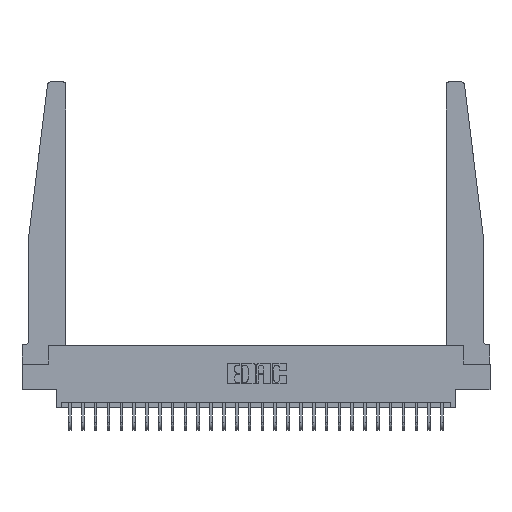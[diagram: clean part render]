
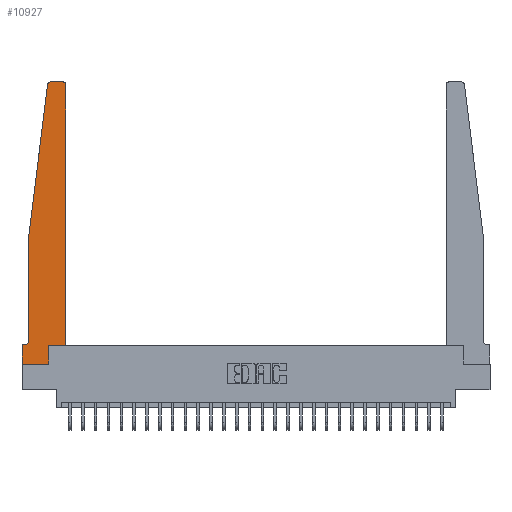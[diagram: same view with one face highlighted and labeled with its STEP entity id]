
A CAD part, top view. The second image highlights one B-rep face of the part: STEP entity #10927.
In plain terms, the highlighted planar face has unit normal (0, 0, 1).
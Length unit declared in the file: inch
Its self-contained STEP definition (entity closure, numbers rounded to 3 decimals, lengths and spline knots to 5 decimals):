
#53 = VERTEX_POINT ( 'NONE', #26011 ) ;
#137 = VERTEX_POINT ( 'NONE', #17653 ) ;
#1219 = VECTOR ( 'NONE', #7749, 39.37008 ) ;
#1226 = VERTEX_POINT ( 'NONE', #22857 ) ;
#1598 = VERTEX_POINT ( 'NONE', #12067 ) ;
#2231 = LINE ( 'NONE', #4086, #17629 ) ;
#2307 = CARTESIAN_POINT ( 'NONE',  ( 0.015, 0.1875, 0.37 ) ) ;
#2978 = CIRCLE ( 'NONE', #25849, 0.05 ) ;
#3392 = PLANE ( 'NONE',  #9828 ) ;
#3404 = VERTEX_POINT ( 'NONE', #27301 ) ;
#3586 = EDGE_CURVE ( 'NONE', #22999, #1226, #22368, .T. ) ;
#3600 = DIRECTION ( 'NONE',  ( 1., 0., 0. ) ) ;
#3619 = VECTOR ( 'NONE', #23617, 39.37008 ) ;
#3697 = LINE ( 'NONE', #27326, #1219 ) ;
#3800 = DIRECTION ( 'NONE',  ( -1., 0., 0. ) ) ;
#3836 = LINE ( 'NONE', #14809, #3619 ) ;
#4086 = CARTESIAN_POINT ( 'NONE',  ( 0.425, 0.18, 0.37 ) ) ;
#4185 = VECTOR ( 'NONE', #24917, 39.37008 ) ;
#4528 = ORIENTED_EDGE ( 'NONE', *, *, #15000, .T. ) ;
#4631 = EDGE_CURVE ( 'NONE', #18367, #1598, #27826, .T. ) ;
#5697 = DIRECTION ( 'NONE',  ( 1., 0., 0. ) ) ;
#6067 = ORIENTED_EDGE ( 'NONE', *, *, #6815, .T. ) ;
#6091 = CARTESIAN_POINT ( 'NONE',  ( 0.395, 2.75, 0.37 ) ) ;
#6325 = AXIS2_PLACEMENT_3D ( 'NONE', #9249, #24589, #13372 ) ;
#6461 = VERTEX_POINT ( 'NONE', #2307 ) ;
#6753 = CARTESIAN_POINT ( 'NONE',  ( 0.425, 2.72, 0.37 ) ) ;
#6815 = EDGE_CURVE ( 'NONE', #137, #22999, #3836, .T. ) ;
#7121 = EDGE_CURVE ( 'NONE', #6461, #137, #12481, .T. ) ;
#7220 = CIRCLE ( 'NONE', #18136, 0.03 ) ;
#7537 = VECTOR ( 'NONE', #11433, 39.37008 ) ;
#7749 = DIRECTION ( 'NONE',  ( 0., -1., 0. ) ) ;
#7797 = CARTESIAN_POINT ( 'NONE',  ( 0.395, 2.72, 0.37 ) ) ;
#7861 = CARTESIAN_POINT ( 'NONE',  ( 0.065, 0.1875, 0.37 ) ) ;
#7934 = DIRECTION ( 'NONE',  ( 0., 1., 0. ) ) ;
#8219 = EDGE_CURVE ( 'NONE', #14300, #6461, #2978, .T. ) ;
#9249 = CARTESIAN_POINT ( 'NONE',  ( 0.27653, 2.72, 0.37 ) ) ;
#9493 = EDGE_CURVE ( 'NONE', #19675, #53, #26091, .T. ) ;
#9828 = AXIS2_PLACEMENT_3D ( 'NONE', #12099, #16811, #5697 ) ;
#10927 = ADVANCED_FACE ( 'NONE', ( #16672 ), #3392, .T. ) ;
#10933 = DIRECTION ( 'NONE',  ( 0., 1., 0. ) ) ;
#10955 = VECTOR ( 'NONE', #7934, 39.37008 ) ;
#11401 = DIRECTION ( 'NONE',  ( -1., 0., 0. ) ) ;
#11433 = DIRECTION ( 'NONE',  ( 1., 0., 0. ) ) ;
#12067 = CARTESIAN_POINT ( 'NONE',  ( 0.27653, 2.75, 0.37 ) ) ;
#12099 = CARTESIAN_POINT ( 'NONE',  ( 0., 0.1875, 0.37 ) ) ;
#12148 = VECTOR ( 'NONE', #15430, 39.37008 ) ;
#12254 = CARTESIAN_POINT ( 'NONE',  ( 0.065, 0.2375, 0.37 ) ) ;
#12349 = ORIENTED_EDGE ( 'NONE', *, *, #27936, .T. ) ;
#12481 = LINE ( 'NONE', #7861, #19610 ) ;
#12694 = ORIENTED_EDGE ( 'NONE', *, *, #3586, .T. ) ;
#13372 = DIRECTION ( 'NONE',  ( 1., 0., 0. ) ) ;
#13546 = CARTESIAN_POINT ( 'NONE',  ( 0.015, 0.2375, 0.37 ) ) ;
#14006 = VERTEX_POINT ( 'NONE', #6753 ) ;
#14189 = LINE ( 'NONE', #16471, #10955 ) ;
#14300 = VERTEX_POINT ( 'NONE', #12254 ) ;
#14666 = ORIENTED_EDGE ( 'NONE', *, *, #20721, .T. ) ;
#14809 = CARTESIAN_POINT ( 'NONE',  ( 0., 0., 0.37 ) ) ;
#14932 = CIRCLE ( 'NONE', #6325, 0.03 ) ;
#15000 = EDGE_CURVE ( 'NONE', #3404, #14006, #2231, .T. ) ;
#15244 = ORIENTED_EDGE ( 'NONE', *, *, #24694, .T. ) ;
#15430 = DIRECTION ( 'NONE',  ( -0.122, -0.992, 0. ) ) ;
#16471 = CARTESIAN_POINT ( 'NONE',  ( 0.2605, 0.18, 0.37 ) ) ;
#16672 = FACE_OUTER_BOUND ( 'NONE', #23894, .T. ) ;
#16811 = DIRECTION ( 'NONE',  ( 0., 0., 1. ) ) ;
#17629 = VECTOR ( 'NONE', #10933, 39.37008 ) ;
#17653 = CARTESIAN_POINT ( 'NONE',  ( 0., 0.1875, 0.37 ) ) ;
#17884 = ORIENTED_EDGE ( 'NONE', *, *, #7121, .T. ) ;
#17987 = CARTESIAN_POINT ( 'NONE',  ( 0.425, 0.18, 0.37 ) ) ;
#18136 = AXIS2_PLACEMENT_3D ( 'NONE', #7797, #23231, #3600 ) ;
#18280 = CARTESIAN_POINT ( 'NONE',  ( 0.25, 2.75, 0.37 ) ) ;
#18291 = DIRECTION ( 'NONE',  ( 1., 0., 0. ) ) ;
#18367 = VERTEX_POINT ( 'NONE', #6091 ) ;
#18896 = ORIENTED_EDGE ( 'NONE', *, *, #4631, .T. ) ;
#19088 = EDGE_CURVE ( 'NONE', #14006, #18367, #7220, .T. ) ;
#19610 = VECTOR ( 'NONE', #3800, 39.37008 ) ;
#19675 = VERTEX_POINT ( 'NONE', #21165 ) ;
#20721 = EDGE_CURVE ( 'NONE', #25146, #3404, #22792, .T. ) ;
#21055 = CARTESIAN_POINT ( 'NONE',  ( 0., 0., 0.37 ) ) ;
#21165 = CARTESIAN_POINT ( 'NONE',  ( 0.24675, 2.72367, 0.37 ) ) ;
#21844 = CARTESIAN_POINT ( 'NONE',  ( 0.2605, 0.18, 0.37 ) ) ;
#22337 = DIRECTION ( 'NONE',  ( 0., 0., -1. ) ) ;
#22368 = LINE ( 'NONE', #26369, #7537 ) ;
#22792 = LINE ( 'NONE', #17987, #25986 ) ;
#22857 = CARTESIAN_POINT ( 'NONE',  ( 0.2605, 0., 0.37 ) ) ;
#22999 = VERTEX_POINT ( 'NONE', #21055 ) ;
#23231 = DIRECTION ( 'NONE',  ( 0., 0., 1. ) ) ;
#23617 = DIRECTION ( 'NONE',  ( 0., -1., 0. ) ) ;
#23661 = EDGE_CURVE ( 'NONE', #1598, #19675, #14932, .T. ) ;
#23894 = EDGE_LOOP ( 'NONE', ( #18896, #28144, #24222, #15244, #28203, #17884, #6067, #12694, #12349, #14666, #4528, #24949 ) ) ;
#24222 = ORIENTED_EDGE ( 'NONE', *, *, #9493, .T. ) ;
#24589 = DIRECTION ( 'NONE',  ( 0., 0., 1. ) ) ;
#24694 = EDGE_CURVE ( 'NONE', #53, #14300, #3697, .T. ) ;
#24917 = DIRECTION ( 'NONE',  ( -1., 0., 0. ) ) ;
#24949 = ORIENTED_EDGE ( 'NONE', *, *, #19088, .T. ) ;
#25146 = VERTEX_POINT ( 'NONE', #21844 ) ;
#25849 = AXIS2_PLACEMENT_3D ( 'NONE', #13546, #22337, #11401 ) ;
#25986 = VECTOR ( 'NONE', #18291, 39.37008 ) ;
#26011 = CARTESIAN_POINT ( 'NONE',  ( 0.065, 1.25, 0.37 ) ) ;
#26091 = LINE ( 'NONE', #28230, #12148 ) ;
#26369 = CARTESIAN_POINT ( 'NONE',  ( 0., 0., 0.37 ) ) ;
#27301 = CARTESIAN_POINT ( 'NONE',  ( 0.425, 0.18, 0.37 ) ) ;
#27326 = CARTESIAN_POINT ( 'NONE',  ( 0.065, 1.25, 0.37 ) ) ;
#27826 = LINE ( 'NONE', #18280, #4185 ) ;
#27936 = EDGE_CURVE ( 'NONE', #1226, #25146, #14189, .T. ) ;
#28144 = ORIENTED_EDGE ( 'NONE', *, *, #23661, .T. ) ;
#28203 = ORIENTED_EDGE ( 'NONE', *, *, #8219, .T. ) ;
#28230 = CARTESIAN_POINT ( 'NONE',  ( 0.065, 1.25, 0.37 ) ) ;
